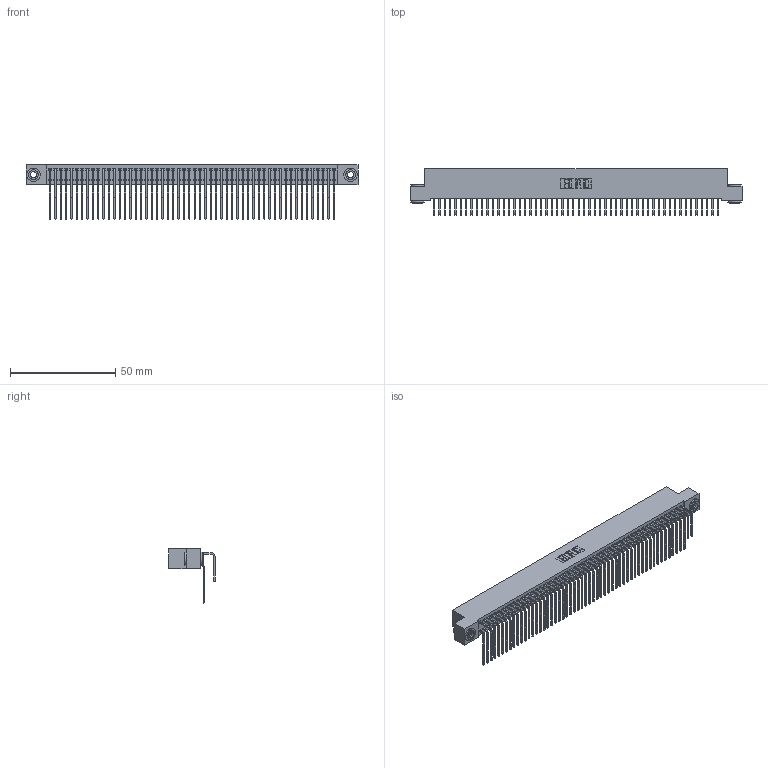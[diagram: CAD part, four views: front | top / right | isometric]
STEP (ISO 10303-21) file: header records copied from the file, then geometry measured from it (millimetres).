
FILE_DESCRIPTION (( 'STEP AP203' ), '1' );
FILE_NAME ('342-108-558-203.STEP', '2019-10-04T19:59:43', ( '' ), ( '' ), 'SwSTEP 2.0', 'SolidWorks 2016', '' );
FILE_SCHEMA (( 'CONFIG_CONTROL_DESIGN' ));
Length unit declared in the file: inch
Products named in the file (5): 345-292-001_558 Tail - 2; 342-250-002_345-250-002-102; 342-108-558-203; 345-292-001_558 559 Tail - 1; 342 Part_.156 TH
Assembly tree (111 placements, depth 2):
  342-108-558-203
    342 Part_.156 TH
    345-292-001_558 559 Tail - 1  x54
    345-292-001_558 Tail - 2  x54
    342-250-002_345-250-002-102  x2
Bounding box: 157.48 x 21.91 x 25.78 mm (x, y, z)
Volume: 14852.2 mm3; surface area: 27503.8 mm2
Topology: 111 solids, 111 shells, 5980 faces, 17763 edges, 11694 vertices
Faces by surface type: plane 4180, cylinder 1792, cone 8
Entity records: 35490 total; most frequent: CARTESIAN_POINT 5892, ORIENTED_EDGE 5770, DIRECTION 5027, EDGE_CURVE 2885, VECTOR 2693, LINE 2693, VERTEX_POINT 1918, AXIS2_PLACEMENT_3D 1167
